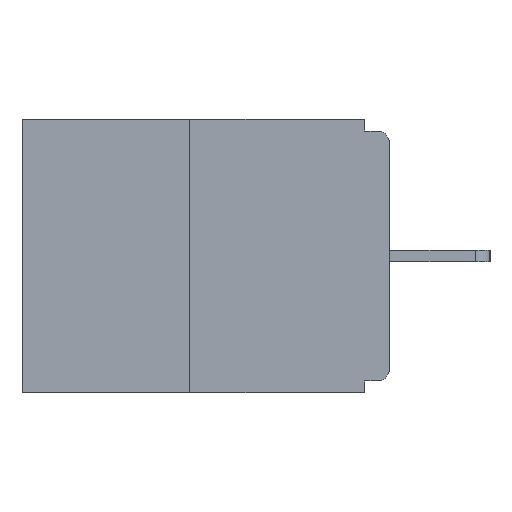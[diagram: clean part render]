
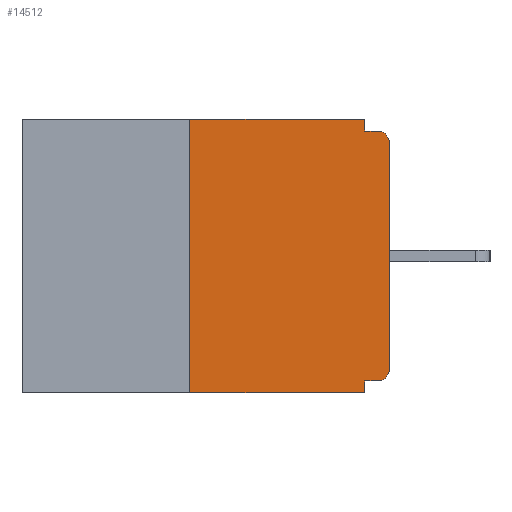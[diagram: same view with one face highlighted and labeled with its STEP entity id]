
A CAD part, left-side view. The second image highlights one B-rep face of the part: STEP entity #14512.
In plain terms, the highlighted planar face has unit normal (-1, 0, 0).
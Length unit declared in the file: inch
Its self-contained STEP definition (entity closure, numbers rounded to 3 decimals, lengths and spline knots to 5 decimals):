
#227 = DIRECTION ( 'NONE',  ( 0., 0., -1. ) ) ;
#408 = EDGE_CURVE ( 'NONE', #541, #9239, #6119, .T. ) ;
#541 = VERTEX_POINT ( 'NONE', #5031 ) ;
#887 = DIRECTION ( 'NONE',  ( 0., 0., -1. ) ) ;
#1011 = VERTEX_POINT ( 'NONE', #16763 ) ;
#1176 = CARTESIAN_POINT ( 'NONE',  ( 0., 0., -0.03 ) ) ;
#1271 = EDGE_CURVE ( 'NONE', #1011, #9098, #18332, .T. ) ;
#1491 = ORIENTED_EDGE ( 'NONE', *, *, #7855, .F. ) ;
#1530 = CARTESIAN_POINT ( 'NONE',  ( 0., 0.46, -0.343 ) ) ;
#1687 = LINE ( 'NONE', #16939, #10647 ) ;
#2361 = VECTOR ( 'NONE', #10612, 39.37008 ) ;
#2652 = DIRECTION ( 'NONE',  ( 0., 0., -1. ) ) ;
#3346 = VERTEX_POINT ( 'NONE', #1176 ) ;
#3957 = PLANE ( 'NONE',  #9264 ) ;
#3963 = CARTESIAN_POINT ( 'NONE',  ( 0., 0.46, 0. ) ) ;
#4278 = VECTOR ( 'NONE', #14480, 39.37008 ) ;
#4434 = ORIENTED_EDGE ( 'NONE', *, *, #12593, .F. ) ;
#4869 = ORIENTED_EDGE ( 'NONE', *, *, #14039, .F. ) ;
#5031 = CARTESIAN_POINT ( 'NONE',  ( 0., 0.015, -0.328 ) ) ;
#5149 = EDGE_CURVE ( 'NONE', #13135, #9098, #20345, .T. ) ;
#5727 = EDGE_CURVE ( 'NONE', #3346, #20472, #10645, .T. ) ;
#5904 = CARTESIAN_POINT ( 'NONE',  ( 0., 0.25, 0. ) ) ;
#6119 = CIRCLE ( 'NONE', #16369, 0.015 ) ;
#6261 = DIRECTION ( 'NONE',  ( 0., 0., -1. ) ) ;
#6320 = CARTESIAN_POINT ( 'NONE',  ( 0., 0., -0.328 ) ) ;
#6523 = EDGE_LOOP ( 'NONE', ( #19276, #1491, #18305, #14187, #4869, #10189, #9520, #9185, #4434, #12660 ) ) ;
#7396 = LINE ( 'NONE', #20691, #2361 ) ;
#7712 = LINE ( 'NONE', #3963, #4278 ) ;
#7855 = EDGE_CURVE ( 'NONE', #1011, #19446, #8138, .T. ) ;
#8138 = LINE ( 'NONE', #9593, #10215 ) ;
#8262 = VECTOR ( 'NONE', #14809, 39.37008 ) ;
#9098 = VERTEX_POINT ( 'NONE', #19247 ) ;
#9185 = ORIENTED_EDGE ( 'NONE', *, *, #5727, .T. ) ;
#9239 = VERTEX_POINT ( 'NONE', #13074 ) ;
#9264 = AXIS2_PLACEMENT_3D ( 'NONE', #10822, #16018, #887 ) ;
#9490 = CARTESIAN_POINT ( 'NONE',  ( 0., 0.031, -0.015 ) ) ;
#9520 = ORIENTED_EDGE ( 'NONE', *, *, #16786, .T. ) ;
#9593 = CARTESIAN_POINT ( 'NONE',  ( 0., 0.25, 0. ) ) ;
#9772 = LINE ( 'NONE', #6320, #10294 ) ;
#10127 = DIRECTION ( 'NONE',  ( 0., 0., -1. ) ) ;
#10173 = VERTEX_POINT ( 'NONE', #17703 ) ;
#10189 = ORIENTED_EDGE ( 'NONE', *, *, #408, .T. ) ;
#10215 = VECTOR ( 'NONE', #16358, 39.37008 ) ;
#10271 = CARTESIAN_POINT ( 'NONE',  ( 0., 0.031, -0.343 ) ) ;
#10294 = VECTOR ( 'NONE', #11446, 39.37008 ) ;
#10612 = DIRECTION ( 'NONE',  ( 0., -1., 0. ) ) ;
#10645 = CIRCLE ( 'NONE', #20847, 0.015 ) ;
#10647 = VECTOR ( 'NONE', #13515, 39.37008 ) ;
#10822 = CARTESIAN_POINT ( 'NONE',  ( 0., 0.46, 0. ) ) ;
#11446 = DIRECTION ( 'NONE',  ( 0., 1., 0. ) ) ;
#11881 = VERTEX_POINT ( 'NONE', #9490 ) ;
#12382 = FACE_OUTER_BOUND ( 'NONE', #6523, .T. ) ;
#12593 = EDGE_CURVE ( 'NONE', #11881, #20472, #7396, .T. ) ;
#12660 = ORIENTED_EDGE ( 'NONE', *, *, #14716, .F. ) ;
#13074 = CARTESIAN_POINT ( 'NONE',  ( 0., 0., -0.313 ) ) ;
#13135 = VERTEX_POINT ( 'NONE', #14594 ) ;
#13515 = DIRECTION ( 'NONE',  ( 0., 0., 1. ) ) ;
#14039 = EDGE_CURVE ( 'NONE', #541, #13135, #9772, .T. ) ;
#14187 = ORIENTED_EDGE ( 'NONE', *, *, #5149, .F. ) ;
#14474 = DIRECTION ( 'NONE',  ( -1., 0., 0. ) ) ;
#14480 = DIRECTION ( 'NONE',  ( 0., -1., 0. ) ) ;
#14512 = ADVANCED_FACE ( 'NONE', ( #12382 ), #3957, .F. ) ;
#14594 = CARTESIAN_POINT ( 'NONE',  ( 0., 0.031, -0.328 ) ) ;
#14716 = EDGE_CURVE ( 'NONE', #10173, #11881, #18862, .T. ) ;
#14809 = DIRECTION ( 'NONE',  ( 0., -1., 0. ) ) ;
#15637 = EDGE_CURVE ( 'NONE', #19446, #10173, #7712, .T. ) ;
#15767 = CARTESIAN_POINT ( 'NONE',  ( 0., 0.015, -0.015 ) ) ;
#16018 = DIRECTION ( 'NONE',  ( 1., 0., 0. ) ) ;
#16343 = CARTESIAN_POINT ( 'NONE',  ( 0., 0.015, -0.313 ) ) ;
#16358 = DIRECTION ( 'NONE',  ( 0., 0., 1. ) ) ;
#16369 = AXIS2_PLACEMENT_3D ( 'NONE', #16343, #21436, #6261 ) ;
#16763 = CARTESIAN_POINT ( 'NONE',  ( 0., 0.25, -0.343 ) ) ;
#16786 = EDGE_CURVE ( 'NONE', #9239, #3346, #1687, .T. ) ;
#16939 = CARTESIAN_POINT ( 'NONE',  ( 0., 0., 0. ) ) ;
#17703 = CARTESIAN_POINT ( 'NONE',  ( 0., 0.031, 0. ) ) ;
#18305 = ORIENTED_EDGE ( 'NONE', *, *, #1271, .T. ) ;
#18332 = LINE ( 'NONE', #1530, #8262 ) ;
#18862 = LINE ( 'NONE', #20517, #19524 ) ;
#18990 = CARTESIAN_POINT ( 'NONE',  ( 0., 0.015, -0.03 ) ) ;
#19247 = CARTESIAN_POINT ( 'NONE',  ( 0., 0.031, -0.343 ) ) ;
#19276 = ORIENTED_EDGE ( 'NONE', *, *, #15637, .F. ) ;
#19302 = VECTOR ( 'NONE', #227, 39.37008 ) ;
#19446 = VERTEX_POINT ( 'NONE', #5904 ) ;
#19524 = VECTOR ( 'NONE', #10127, 39.37008 ) ;
#20345 = LINE ( 'NONE', #10271, #19302 ) ;
#20472 = VERTEX_POINT ( 'NONE', #15767 ) ;
#20517 = CARTESIAN_POINT ( 'NONE',  ( 0., 0.031, 0. ) ) ;
#20691 = CARTESIAN_POINT ( 'NONE',  ( 0., 0., -0.015 ) ) ;
#20847 = AXIS2_PLACEMENT_3D ( 'NONE', #18990, #14474, #2652 ) ;
#21436 = DIRECTION ( 'NONE',  ( -1., 0., 0. ) ) ;
